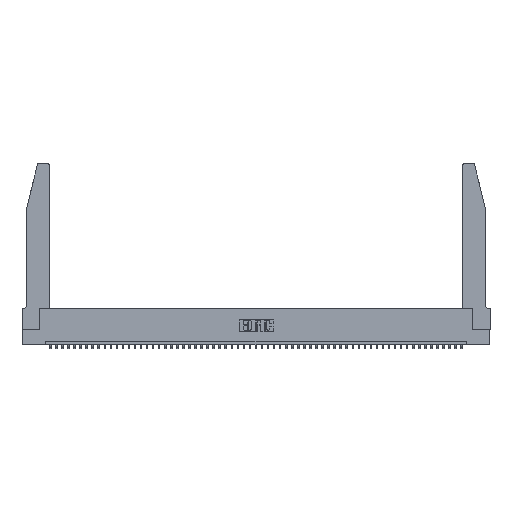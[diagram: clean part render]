
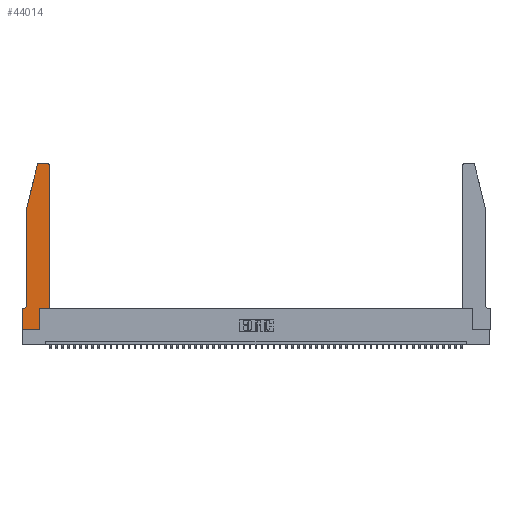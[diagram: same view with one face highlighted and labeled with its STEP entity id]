
A CAD part, top view. The second image highlights one B-rep face of the part: STEP entity #44014.
In plain terms, the highlighted planar face has unit normal (0, 0, 1).
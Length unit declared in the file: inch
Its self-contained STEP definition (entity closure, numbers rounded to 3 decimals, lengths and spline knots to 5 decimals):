
#353 = LINE ( 'NONE', #6158, #51639 ) ;
#371 = CARTESIAN_POINT ( 'NONE',  ( 0., 0., 0.37 ) ) ;
#419 = EDGE_CURVE ( 'NONE', #7193, #52328, #10820, .T. ) ;
#555 = ORIENTED_EDGE ( 'NONE', *, *, #25522, .T. ) ;
#1385 = CARTESIAN_POINT ( 'NONE',  ( 0.2865, 0.35, 0.37 ) ) ;
#1584 = DIRECTION ( 'NONE',  ( 0., 1., 0. ) ) ;
#2216 = DIRECTION ( 'NONE',  ( -1., 0., 0. ) ) ;
#2245 = ORIENTED_EDGE ( 'NONE', *, *, #47614, .T. ) ;
#3404 = CARTESIAN_POINT ( 'NONE',  ( 0.4505, 2.72, 0.37 ) ) ;
#4406 = CIRCLE ( 'NONE', #14474, 0.07 ) ;
#5907 = CARTESIAN_POINT ( 'NONE',  ( 0.284, 2.75, 0.37 ) ) ;
#6053 = DIRECTION ( 'NONE',  ( -1., 0., 0. ) ) ;
#6158 = CARTESIAN_POINT ( 'NONE',  ( 0.0755, 0.35, 0.37 ) ) ;
#6954 = EDGE_CURVE ( 'NONE', #48946, #20723, #35316, .T. ) ;
#7193 = VERTEX_POINT ( 'NONE', #28066 ) ;
#8649 = CARTESIAN_POINT ( 'NONE',  ( 0.0755, 0.42, 0.37 ) ) ;
#8842 = LINE ( 'NONE', #13945, #37722 ) ;
#9995 = LINE ( 'NONE', #25548, #24156 ) ;
#10820 = LINE ( 'NONE', #22238, #33890 ) ;
#11314 = CIRCLE ( 'NONE', #34295, 0.03 ) ;
#11572 = DIRECTION ( 'NONE',  ( 0., 0., 1. ) ) ;
#11632 = VECTOR ( 'NONE', #32356, 39.37008 ) ;
#12771 = VERTEX_POINT ( 'NONE', #16038 ) ;
#13234 = EDGE_CURVE ( 'NONE', #45198, #12771, #4406, .T. ) ;
#13640 = VERTEX_POINT ( 'NONE', #38074 ) ;
#13945 = CARTESIAN_POINT ( 'NONE',  ( 0.2865, 0.35, 0.37 ) ) ;
#14424 = VERTEX_POINT ( 'NONE', #16058 ) ;
#14474 = AXIS2_PLACEMENT_3D ( 'NONE', #30660, #47682, #47496 ) ;
#15347 = CARTESIAN_POINT ( 'NONE',  ( 0.0755, 2., 0.37 ) ) ;
#15739 = ORIENTED_EDGE ( 'NONE', *, *, #21067, .T. ) ;
#16038 = CARTESIAN_POINT ( 'NONE',  ( 0.0055, 0.35, 0.37 ) ) ;
#16058 = CARTESIAN_POINT ( 'NONE',  ( 0.2865, 0., 0.37 ) ) ;
#16507 = ORIENTED_EDGE ( 'NONE', *, *, #17339, .T. ) ;
#17339 = EDGE_CURVE ( 'NONE', #52328, #35728, #44418, .T. ) ;
#19785 = EDGE_CURVE ( 'NONE', #38356, #13640, #48737, .T. ) ;
#20190 = CARTESIAN_POINT ( 'NONE',  ( 0., 0.35, 0.37 ) ) ;
#20341 = LINE ( 'NONE', #371, #50466 ) ;
#20723 = VERTEX_POINT ( 'NONE', #47516 ) ;
#21067 = EDGE_CURVE ( 'NONE', #20723, #14424, #20341, .T. ) ;
#21543 = LINE ( 'NONE', #45748, #38801 ) ;
#21943 = VERTEX_POINT ( 'NONE', #42433 ) ;
#22238 = CARTESIAN_POINT ( 'NONE',  ( 0.2605, 2.75, 0.37 ) ) ;
#22651 = CARTESIAN_POINT ( 'NONE',  ( 0.4505, 0.35, 0.37 ) ) ;
#22664 = ORIENTED_EDGE ( 'NONE', *, *, #19785, .T. ) ;
#24155 = DIRECTION ( 'NONE',  ( 0., -1., 0. ) ) ;
#24156 = VECTOR ( 'NONE', #46353, 39.37008 ) ;
#24558 = CARTESIAN_POINT ( 'NONE',  ( 0.4205, 2.72, 0.37 ) ) ;
#24571 = ORIENTED_EDGE ( 'NONE', *, *, #25174, .T. ) ;
#24676 = ORIENTED_EDGE ( 'NONE', *, *, #25063, .T. ) ;
#24887 = VERTEX_POINT ( 'NONE', #3404 ) ;
#25063 = EDGE_CURVE ( 'NONE', #13640, #24887, #9995, .T. ) ;
#25174 = EDGE_CURVE ( 'NONE', #24887, #7193, #11314, .T. ) ;
#25522 = EDGE_CURVE ( 'NONE', #12771, #48946, #353, .T. ) ;
#25548 = CARTESIAN_POINT ( 'NONE',  ( 0.4505, 0.35, 0.37 ) ) ;
#25774 = DIRECTION ( 'NONE',  ( 1., 0., 0. ) ) ;
#26284 = ORIENTED_EDGE ( 'NONE', *, *, #35619, .T. ) ;
#27644 = AXIS2_PLACEMENT_3D ( 'NONE', #20190, #11572, #52811 ) ;
#28066 = CARTESIAN_POINT ( 'NONE',  ( 0.4205, 2.75, 0.37 ) ) ;
#30216 = ORIENTED_EDGE ( 'NONE', *, *, #6954, .T. ) ;
#30660 = CARTESIAN_POINT ( 'NONE',  ( 0.0055, 0.42, 0.37 ) ) ;
#32356 = DIRECTION ( 'NONE',  ( 0., -1., 0. ) ) ;
#33890 = VECTOR ( 'NONE', #6053, 39.37008 ) ;
#34295 = AXIS2_PLACEMENT_3D ( 'NONE', #24558, #53041, #37082 ) ;
#34367 = CARTESIAN_POINT ( 'NONE',  ( 0.284, 2.72, 0.37 ) ) ;
#35316 = LINE ( 'NONE', #52070, #11632 ) ;
#35619 = EDGE_CURVE ( 'NONE', #35728, #21943, #21543, .T. ) ;
#35728 = VERTEX_POINT ( 'NONE', #42249 ) ;
#35883 = VECTOR ( 'NONE', #38588, 39.37008 ) ;
#37082 = DIRECTION ( 'NONE',  ( 1., 0., 0. ) ) ;
#37722 = VECTOR ( 'NONE', #1584, 39.37008 ) ;
#38074 = CARTESIAN_POINT ( 'NONE',  ( 0.4505, 0.35, 0.37 ) ) ;
#38356 = VERTEX_POINT ( 'NONE', #1385 ) ;
#38588 = DIRECTION ( 'NONE',  ( 1., 0., 0. ) ) ;
#38723 = EDGE_LOOP ( 'NONE', ( #52465, #16507, #26284, #2245, #47838, #555, #30216, #15739, #44528, #22664, #24676, #24571 ) ) ;
#38801 = VECTOR ( 'NONE', #49507, 39.37008 ) ;
#39519 = LINE ( 'NONE', #15347, #42691 ) ;
#40032 = PLANE ( 'NONE',  #27644 ) ;
#41378 = DIRECTION ( 'NONE',  ( 1., 0., 0. ) ) ;
#42213 = DIRECTION ( 'NONE',  ( 0., 0., 1. ) ) ;
#42249 = CARTESIAN_POINT ( 'NONE',  ( 0.25487, 2.72718, 0.37 ) ) ;
#42433 = CARTESIAN_POINT ( 'NONE',  ( 0.0755, 2., 0.37 ) ) ;
#42691 = VECTOR ( 'NONE', #24155, 39.37008 ) ;
#44014 = ADVANCED_FACE ( 'NONE', ( #52145 ), #40032, .T. ) ;
#44418 = CIRCLE ( 'NONE', #49019, 0.03 ) ;
#44528 = ORIENTED_EDGE ( 'NONE', *, *, #52901, .T. ) ;
#45198 = VERTEX_POINT ( 'NONE', #8649 ) ;
#45748 = CARTESIAN_POINT ( 'NONE',  ( 0.0755, 2., 0.37 ) ) ;
#46353 = DIRECTION ( 'NONE',  ( 0., 1., 0. ) ) ;
#47496 = DIRECTION ( 'NONE',  ( -1., 0., 0. ) ) ;
#47516 = CARTESIAN_POINT ( 'NONE',  ( 0., 0., 0.37 ) ) ;
#47614 = EDGE_CURVE ( 'NONE', #21943, #45198, #39519, .T. ) ;
#47682 = DIRECTION ( 'NONE',  ( 0., 0., -1. ) ) ;
#47838 = ORIENTED_EDGE ( 'NONE', *, *, #13234, .T. ) ;
#48737 = LINE ( 'NONE', #22651, #35883 ) ;
#48946 = VERTEX_POINT ( 'NONE', #53030 ) ;
#49019 = AXIS2_PLACEMENT_3D ( 'NONE', #34367, #42213, #25774 ) ;
#49507 = DIRECTION ( 'NONE',  ( -0.239, -0.971, 0. ) ) ;
#50466 = VECTOR ( 'NONE', #41378, 39.37008 ) ;
#51639 = VECTOR ( 'NONE', #2216, 39.37008 ) ;
#52070 = CARTESIAN_POINT ( 'NONE',  ( 0., 0., 0.37 ) ) ;
#52145 = FACE_OUTER_BOUND ( 'NONE', #38723, .T. ) ;
#52328 = VERTEX_POINT ( 'NONE', #5907 ) ;
#52465 = ORIENTED_EDGE ( 'NONE', *, *, #419, .T. ) ;
#52811 = DIRECTION ( 'NONE',  ( 1., 0., 0. ) ) ;
#52901 = EDGE_CURVE ( 'NONE', #14424, #38356, #8842, .T. ) ;
#53030 = CARTESIAN_POINT ( 'NONE',  ( 0., 0.35, 0.37 ) ) ;
#53041 = DIRECTION ( 'NONE',  ( 0., 0., 1. ) ) ;
